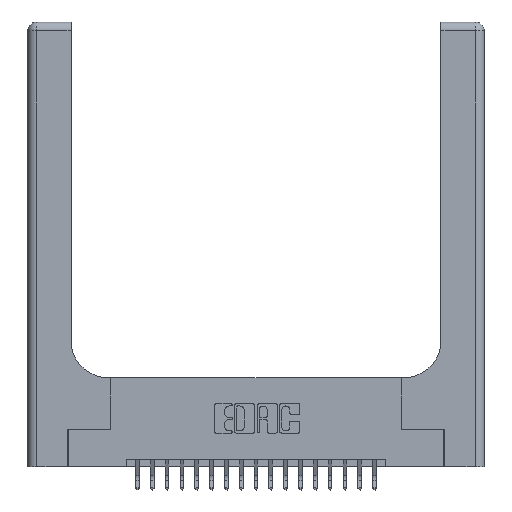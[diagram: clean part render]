
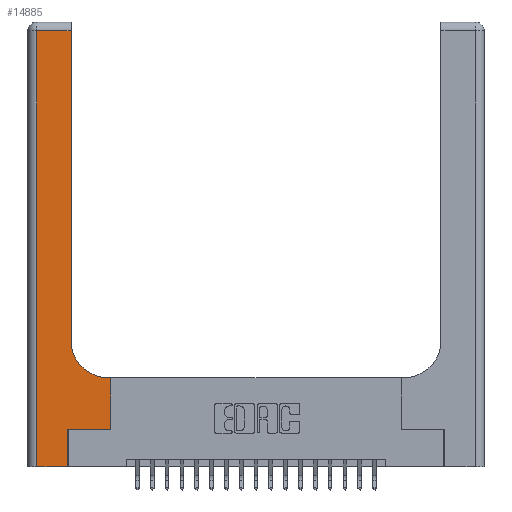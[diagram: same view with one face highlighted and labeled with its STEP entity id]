
A CAD part, top view. The second image highlights one B-rep face of the part: STEP entity #14885.
In plain terms, the highlighted planar face has unit normal (0, 0, 1).
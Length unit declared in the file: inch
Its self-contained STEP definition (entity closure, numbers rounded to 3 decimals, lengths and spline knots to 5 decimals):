
#252 = VECTOR ( 'NONE', #4269, 39.37008 ) ;
#424 = VECTOR ( 'NONE', #14171, 39.37008 ) ;
#478 = DIRECTION ( 'NONE',  ( 1., 0., 0. ) ) ;
#750 = CARTESIAN_POINT ( 'NONE',  ( 0.2915, 0.6, 0.37 ) ) ;
#774 = LINE ( 'NONE', #5336, #5849 ) ;
#1029 = EDGE_LOOP ( 'NONE', ( #7428, #7194, #17081, #3273, #1240, #2246, #2367, #17977, #1896 ) ) ;
#1240 = ORIENTED_EDGE ( 'NONE', *, *, #15883, .T. ) ;
#1765 = LINE ( 'NONE', #5839, #20244 ) ;
#1877 = VECTOR ( 'NONE', #15583, 39.37008 ) ;
#1896 = ORIENTED_EDGE ( 'NONE', *, *, #13279, .T. ) ;
#2246 = ORIENTED_EDGE ( 'NONE', *, *, #3264, .T. ) ;
#2367 = ORIENTED_EDGE ( 'NONE', *, *, #11820, .T. ) ;
#2474 = CARTESIAN_POINT ( 'NONE',  ( 0.269, 0., 0.37 ) ) ;
#3022 = DIRECTION ( 'NONE',  ( 1., 0., 0. ) ) ;
#3264 = EDGE_CURVE ( 'NONE', #21401, #9192, #21144, .T. ) ;
#3273 = ORIENTED_EDGE ( 'NONE', *, *, #15761, .T. ) ;
#4269 = DIRECTION ( 'NONE',  ( 0., 1., 0. ) ) ;
#4431 = FACE_OUTER_BOUND ( 'NONE', #1029, .T. ) ;
#4456 = VERTEX_POINT ( 'NONE', #12613 ) ;
#5157 = VECTOR ( 'NONE', #14186, 39.37008 ) ;
#5336 = CARTESIAN_POINT ( 'NONE',  ( 0., 2.94, 0.37 ) ) ;
#5568 = CARTESIAN_POINT ( 'NONE',  ( 0.5415, 0.6, 0.37 ) ) ;
#5839 = CARTESIAN_POINT ( 'NONE',  ( 0.06, 3., 0.37 ) ) ;
#5849 = VECTOR ( 'NONE', #18953, 39.37008 ) ;
#5966 = DIRECTION ( 'NONE',  ( 0., 0., -1. ) ) ;
#6419 = CARTESIAN_POINT ( 'NONE',  ( 0.269, 0.25, 0.37 ) ) ;
#6543 = EDGE_CURVE ( 'NONE', #6791, #16499, #1765, .T. ) ;
#6791 = VERTEX_POINT ( 'NONE', #15967 ) ;
#7194 = ORIENTED_EDGE ( 'NONE', *, *, #20530, .T. ) ;
#7428 = ORIENTED_EDGE ( 'NONE', *, *, #10156, .T. ) ;
#7488 = LINE ( 'NONE', #2474, #252 ) ;
#8455 = CARTESIAN_POINT ( 'NONE',  ( 0.2915, 2.94, 0.37 ) ) ;
#8891 = CARTESIAN_POINT ( 'NONE',  ( 0.5585, 0.25, 0.37 ) ) ;
#8898 = LINE ( 'NONE', #10760, #5157 ) ;
#9062 = AXIS2_PLACEMENT_3D ( 'NONE', #9981, #16706, #3022 ) ;
#9192 = VERTEX_POINT ( 'NONE', #9478 ) ;
#9478 = CARTESIAN_POINT ( 'NONE',  ( 0.5585, 0.25, 0.37 ) ) ;
#9981 = CARTESIAN_POINT ( 'NONE',  ( 0.5415, 0.85, 0.37 ) ) ;
#10156 = EDGE_CURVE ( 'NONE', #4456, #14518, #8898, .T. ) ;
#10242 = VERTEX_POINT ( 'NONE', #14729 ) ;
#10760 = CARTESIAN_POINT ( 'NONE',  ( 0.2915, 3., 0.37 ) ) ;
#11148 = CIRCLE ( 'NONE', #9062, 0.25 ) ;
#11178 = PLANE ( 'NONE',  #16373 ) ;
#11343 = CARTESIAN_POINT ( 'NONE',  ( 0.06, 0., 0.37 ) ) ;
#11820 = EDGE_CURVE ( 'NONE', #9192, #13551, #14168, .T. ) ;
#12063 = VECTOR ( 'NONE', #19917, 39.37008 ) ;
#12613 = CARTESIAN_POINT ( 'NONE',  ( 0.2915, 0.85, 0.37 ) ) ;
#13097 = LINE ( 'NONE', #16007, #17109 ) ;
#13279 = EDGE_CURVE ( 'NONE', #18638, #4456, #11148, .T. ) ;
#13551 = VERTEX_POINT ( 'NONE', #17979 ) ;
#14168 = LINE ( 'NONE', #8891, #1877 ) ;
#14171 = DIRECTION ( 'NONE',  ( -1., 0., 0. ) ) ;
#14186 = DIRECTION ( 'NONE',  ( 0., 1., 0. ) ) ;
#14518 = VERTEX_POINT ( 'NONE', #8455 ) ;
#14729 = CARTESIAN_POINT ( 'NONE',  ( 0.269, 0., 0.37 ) ) ;
#14743 = EDGE_CURVE ( 'NONE', #13551, #18638, #14861, .T. ) ;
#14861 = LINE ( 'NONE', #750, #424 ) ;
#14885 = ADVANCED_FACE ( 'NONE', ( #4431 ), #11178, .F. ) ;
#15583 = DIRECTION ( 'NONE',  ( 0., 1., 0. ) ) ;
#15761 = EDGE_CURVE ( 'NONE', #16499, #10242, #13097, .T. ) ;
#15883 = EDGE_CURVE ( 'NONE', #10242, #21401, #7488, .T. ) ;
#15967 = CARTESIAN_POINT ( 'NONE',  ( 0.06, 2.94, 0.37 ) ) ;
#16007 = CARTESIAN_POINT ( 'NONE',  ( 0., 0., 0.37 ) ) ;
#16187 = CARTESIAN_POINT ( 'NONE',  ( 0., 3., 0.37 ) ) ;
#16373 = AXIS2_PLACEMENT_3D ( 'NONE', #16187, #5966, #18072 ) ;
#16499 = VERTEX_POINT ( 'NONE', #11343 ) ;
#16706 = DIRECTION ( 'NONE',  ( 0., 0., -1. ) ) ;
#17081 = ORIENTED_EDGE ( 'NONE', *, *, #6543, .T. ) ;
#17109 = VECTOR ( 'NONE', #478, 39.37008 ) ;
#17656 = CARTESIAN_POINT ( 'NONE',  ( 0.269, 0.25, 0.37 ) ) ;
#17786 = DIRECTION ( 'NONE',  ( 0., -1., 0. ) ) ;
#17977 = ORIENTED_EDGE ( 'NONE', *, *, #14743, .T. ) ;
#17979 = CARTESIAN_POINT ( 'NONE',  ( 0.5585, 0.6, 0.37 ) ) ;
#18072 = DIRECTION ( 'NONE',  ( -1., 0., 0. ) ) ;
#18638 = VERTEX_POINT ( 'NONE', #5568 ) ;
#18953 = DIRECTION ( 'NONE',  ( -1., 0., 0. ) ) ;
#19917 = DIRECTION ( 'NONE',  ( 1., 0., 0. ) ) ;
#20244 = VECTOR ( 'NONE', #17786, 39.37008 ) ;
#20530 = EDGE_CURVE ( 'NONE', #14518, #6791, #774, .T. ) ;
#21144 = LINE ( 'NONE', #17656, #12063 ) ;
#21401 = VERTEX_POINT ( 'NONE', #6419 ) ;
